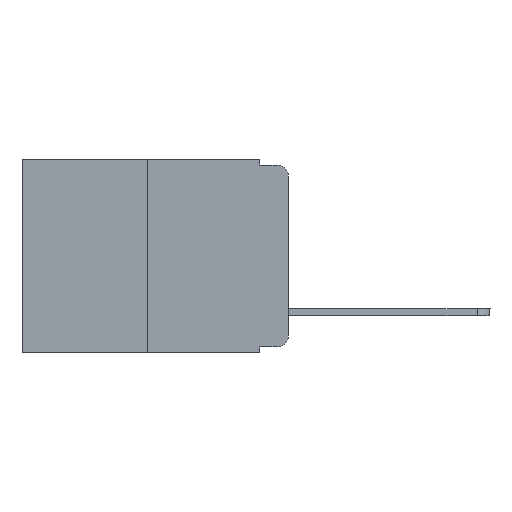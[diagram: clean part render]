
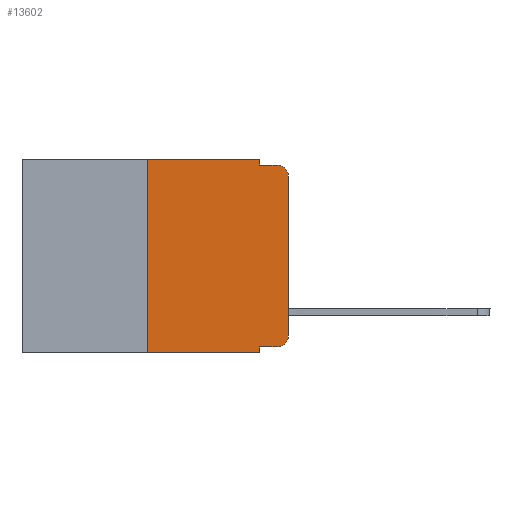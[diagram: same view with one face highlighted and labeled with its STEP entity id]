
A CAD part, left-side view. The second image highlights one B-rep face of the part: STEP entity #13602.
In plain terms, the highlighted planar face has unit normal (-1, 0, 0).
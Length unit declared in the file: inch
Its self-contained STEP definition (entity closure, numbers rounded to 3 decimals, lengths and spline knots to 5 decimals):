
#166 = VECTOR ( 'NONE', #22684, 39.37008 ) ;
#647 = ORIENTED_EDGE ( 'NONE', *, *, #14766, .F. ) ;
#1412 = LINE ( 'NONE', #12931, #166 ) ;
#1581 = DIRECTION ( 'NONE',  ( 0., 0., -1. ) ) ;
#2058 = EDGE_CURVE ( 'NONE', #17208, #14487, #10956, .T. ) ;
#2326 = ORIENTED_EDGE ( 'NONE', *, *, #8037, .F. ) ;
#2519 = VERTEX_POINT ( 'NONE', #23694 ) ;
#2557 = DIRECTION ( 'NONE',  ( 0., 0., 1. ) ) ;
#3251 = ORIENTED_EDGE ( 'NONE', *, *, #9867, .T. ) ;
#3584 = CARTESIAN_POINT ( 'NONE',  ( 0., 0.473, -0.343 ) ) ;
#3668 = VECTOR ( 'NONE', #4938, 39.37008 ) ;
#3827 = ORIENTED_EDGE ( 'NONE', *, *, #14316, .F. ) ;
#4536 = CARTESIAN_POINT ( 'NONE',  ( 0., 0., -0.313 ) ) ;
#4938 = DIRECTION ( 'NONE',  ( 0., -1., 0. ) ) ;
#5193 = LINE ( 'NONE', #3584, #16279 ) ;
#5324 = CARTESIAN_POINT ( 'NONE',  ( 0., 0.051, 0. ) ) ;
#5425 = CARTESIAN_POINT ( 'NONE',  ( 0., 0.051, -0.333 ) ) ;
#5893 = DIRECTION ( 'NONE',  ( 1., 0., 0. ) ) ;
#6290 = CARTESIAN_POINT ( 'NONE',  ( 0., 0.051, -0.343 ) ) ;
#6352 = VECTOR ( 'NONE', #15287, 39.37008 ) ;
#6565 = ORIENTED_EDGE ( 'NONE', *, *, #20048, .T. ) ;
#6856 = LINE ( 'NONE', #11358, #19430 ) ;
#7207 = AXIS2_PLACEMENT_3D ( 'NONE', #19557, #9378, #1581 ) ;
#7253 = CARTESIAN_POINT ( 'NONE',  ( 0., 0., -0.03 ) ) ;
#7599 = CARTESIAN_POINT ( 'NONE',  ( 0., 0.051, -0.01 ) ) ;
#7614 = ORIENTED_EDGE ( 'NONE', *, *, #2058, .T. ) ;
#7945 = DIRECTION ( 'NONE',  ( 0., 0., 1. ) ) ;
#8037 = EDGE_CURVE ( 'NONE', #2519, #9824, #13797, .T. ) ;
#8126 = VERTEX_POINT ( 'NONE', #6290 ) ;
#8613 = ORIENTED_EDGE ( 'NONE', *, *, #18432, .T. ) ;
#8971 = CIRCLE ( 'NONE', #7207, 0.02 ) ;
#9345 = EDGE_CURVE ( 'NONE', #12636, #21921, #11605, .T. ) ;
#9378 = DIRECTION ( 'NONE',  ( -1., 0., 0. ) ) ;
#9403 = DIRECTION ( 'NONE',  ( 0., 0., -1. ) ) ;
#9824 = VERTEX_POINT ( 'NONE', #15890 ) ;
#9867 = EDGE_CURVE ( 'NONE', #24486, #13023, #8971, .T. ) ;
#9868 = CARTESIAN_POINT ( 'NONE',  ( 0., 0.473, 0. ) ) ;
#10177 = CARTESIAN_POINT ( 'NONE',  ( 0., 0.051, 0. ) ) ;
#10597 = DIRECTION ( 'NONE',  ( 0., 0., -1. ) ) ;
#10712 = CARTESIAN_POINT ( 'NONE',  ( 0., 0.051, -0.333 ) ) ;
#10956 = CIRCLE ( 'NONE', #20527, 0.02 ) ;
#11358 = CARTESIAN_POINT ( 'NONE',  ( 0., 0.051, 0. ) ) ;
#11419 = DIRECTION ( 'NONE',  ( 0., -1., 0. ) ) ;
#11605 = LINE ( 'NONE', #5324, #6352 ) ;
#12404 = LINE ( 'NONE', #18056, #13020 ) ;
#12448 = DIRECTION ( 'NONE',  ( -1., 0., 0. ) ) ;
#12532 = LINE ( 'NONE', #20038, #13458 ) ;
#12636 = VERTEX_POINT ( 'NONE', #10177 ) ;
#12931 = CARTESIAN_POINT ( 'NONE',  ( 0., 0.051, -0.01 ) ) ;
#13020 = VECTOR ( 'NONE', #20021, 39.37008 ) ;
#13023 = VERTEX_POINT ( 'NONE', #4536 ) ;
#13458 = VECTOR ( 'NONE', #2557, 39.37008 ) ;
#13602 = ADVANCED_FACE ( 'NONE', ( #21052 ), #15178, .F. ) ;
#13793 = LINE ( 'NONE', #10712, #3668 ) ;
#13797 = LINE ( 'NONE', #21640, #20226 ) ;
#14316 = EDGE_CURVE ( 'NONE', #21921, #14487, #1412, .T. ) ;
#14487 = VERTEX_POINT ( 'NONE', #15346 ) ;
#14536 = ORIENTED_EDGE ( 'NONE', *, *, #20781, .T. ) ;
#14766 = EDGE_CURVE ( 'NONE', #9824, #12636, #12404, .T. ) ;
#15178 = PLANE ( 'NONE',  #16299 ) ;
#15287 = DIRECTION ( 'NONE',  ( 0., 0., -1. ) ) ;
#15346 = CARTESIAN_POINT ( 'NONE',  ( 0., 0.02, -0.01 ) ) ;
#15890 = CARTESIAN_POINT ( 'NONE',  ( 0., 0.25, 0. ) ) ;
#16210 = VERTEX_POINT ( 'NONE', #5425 ) ;
#16279 = VECTOR ( 'NONE', #11419, 39.37008 ) ;
#16291 = EDGE_CURVE ( 'NONE', #16210, #8126, #6856, .T. ) ;
#16299 = AXIS2_PLACEMENT_3D ( 'NONE', #9868, #5893, #25343 ) ;
#17208 = VERTEX_POINT ( 'NONE', #7253 ) ;
#18056 = CARTESIAN_POINT ( 'NONE',  ( 0., 0.473, 0. ) ) ;
#18288 = CARTESIAN_POINT ( 'NONE',  ( 0., 0.02, -0.03 ) ) ;
#18432 = EDGE_CURVE ( 'NONE', #2519, #8126, #5193, .T. ) ;
#19430 = VECTOR ( 'NONE', #9403, 39.37008 ) ;
#19557 = CARTESIAN_POINT ( 'NONE',  ( 0., 0.02, -0.313 ) ) ;
#20021 = DIRECTION ( 'NONE',  ( 0., -1., 0. ) ) ;
#20038 = CARTESIAN_POINT ( 'NONE',  ( 0., 0., 0. ) ) ;
#20048 = EDGE_CURVE ( 'NONE', #16210, #24486, #13793, .T. ) ;
#20226 = VECTOR ( 'NONE', #7945, 39.37008 ) ;
#20527 = AXIS2_PLACEMENT_3D ( 'NONE', #18288, #12448, #10597 ) ;
#20781 = EDGE_CURVE ( 'NONE', #13023, #17208, #12532, .T. ) ;
#21052 = FACE_OUTER_BOUND ( 'NONE', #22795, .T. ) ;
#21186 = ORIENTED_EDGE ( 'NONE', *, *, #9345, .F. ) ;
#21640 = CARTESIAN_POINT ( 'NONE',  ( 0., 0.25, 0. ) ) ;
#21921 = VERTEX_POINT ( 'NONE', #7599 ) ;
#22684 = DIRECTION ( 'NONE',  ( 0., -1., 0. ) ) ;
#22795 = EDGE_LOOP ( 'NONE', ( #14536, #7614, #3827, #21186, #647, #2326, #8613, #24506, #6565, #3251 ) ) ;
#23694 = CARTESIAN_POINT ( 'NONE',  ( 0., 0.25, -0.343 ) ) ;
#24289 = CARTESIAN_POINT ( 'NONE',  ( 0., 0.02, -0.333 ) ) ;
#24486 = VERTEX_POINT ( 'NONE', #24289 ) ;
#24506 = ORIENTED_EDGE ( 'NONE', *, *, #16291, .F. ) ;
#25343 = DIRECTION ( 'NONE',  ( 0., 0., -1. ) ) ;
